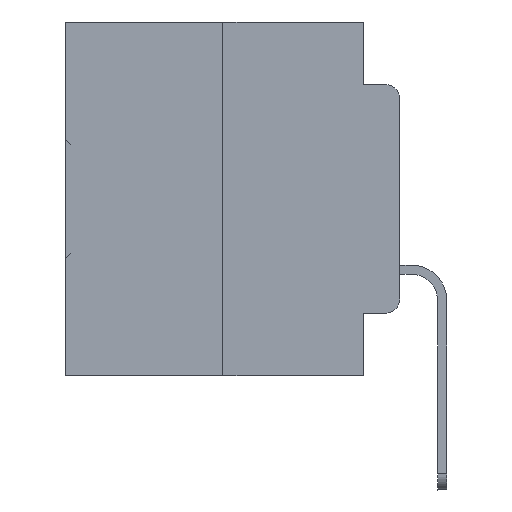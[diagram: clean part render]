
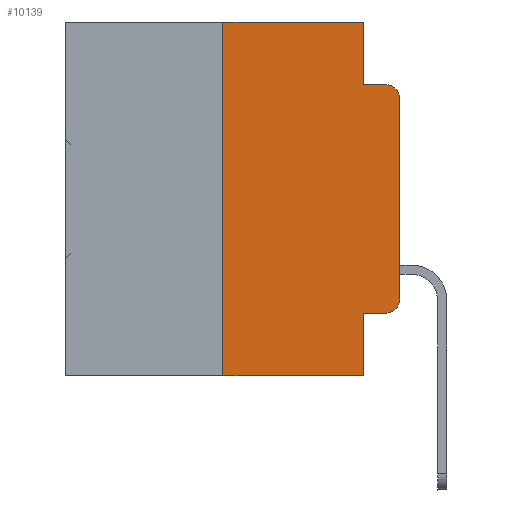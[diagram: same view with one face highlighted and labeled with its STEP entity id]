
A CAD part, left-side view. The second image highlights one B-rep face of the part: STEP entity #10139.
In plain terms, the highlighted planar face has unit normal (-1, 0, 0).
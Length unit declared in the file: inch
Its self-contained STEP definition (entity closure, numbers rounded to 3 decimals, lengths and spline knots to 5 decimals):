
#344 = VERTEX_POINT ( 'NONE', #29676 ) ;
#1409 = EDGE_CURVE ( 'NONE', #12813, #31002, #32425, .T. ) ;
#1522 = CARTESIAN_POINT ( 'NONE',  ( 0., 0., 0. ) ) ;
#1633 = CARTESIAN_POINT ( 'NONE',  ( 0., 0.051, -0.0885 ) ) ;
#2206 = LINE ( 'NONE', #34724, #25309 ) ;
#2281 = CARTESIAN_POINT ( 'NONE',  ( 0., 0.051, -0.4115 ) ) ;
#2851 = CARTESIAN_POINT ( 'NONE',  ( 0., 0.02, -0.1085 ) ) ;
#3725 = CARTESIAN_POINT ( 'NONE',  ( 0., 0.473, -0.5 ) ) ;
#4176 = CARTESIAN_POINT ( 'NONE',  ( 0., 0.02, -0.0885 ) ) ;
#4238 = PLANE ( 'NONE',  #6801 ) ;
#4602 = DIRECTION ( 'NONE',  ( 0., 0., -1. ) ) ;
#4656 = VECTOR ( 'NONE', #28134, 39.37008 ) ;
#5333 = DIRECTION ( 'NONE',  ( 0., 0., -1. ) ) ;
#5848 = EDGE_CURVE ( 'NONE', #8523, #9873, #6689, .T. ) ;
#6689 = LINE ( 'NONE', #14705, #17025 ) ;
#6700 = VECTOR ( 'NONE', #32070, 39.37008 ) ;
#6801 = AXIS2_PLACEMENT_3D ( 'NONE', #12415, #17924, #4602 ) ;
#7383 = LINE ( 'NONE', #1522, #31598 ) ;
#7455 = DIRECTION ( 'NONE',  ( -1., 0., 0. ) ) ;
#8523 = VERTEX_POINT ( 'NONE', #9254 ) ;
#9254 = CARTESIAN_POINT ( 'NONE',  ( 0., 0.051, 0. ) ) ;
#9873 = VERTEX_POINT ( 'NONE', #26986 ) ;
#9907 = CARTESIAN_POINT ( 'NONE',  ( 0., 0.473, 0. ) ) ;
#10139 = ADVANCED_FACE ( 'NONE', ( #28576 ), #4238, .F. ) ;
#10294 = CIRCLE ( 'NONE', #30708, 0.02 ) ;
#11257 = ORIENTED_EDGE ( 'NONE', *, *, #5848, .F. ) ;
#11300 = ORIENTED_EDGE ( 'NONE', *, *, #24654, .T. ) ;
#11871 = VERTEX_POINT ( 'NONE', #15208 ) ;
#12247 = ORIENTED_EDGE ( 'NONE', *, *, #19161, .F. ) ;
#12415 = CARTESIAN_POINT ( 'NONE',  ( 0., 0.473, 0. ) ) ;
#12483 = LINE ( 'NONE', #1633, #19912 ) ;
#12813 = VERTEX_POINT ( 'NONE', #2281 ) ;
#13400 = CARTESIAN_POINT ( 'NONE',  ( 0., 0.02, -0.4115 ) ) ;
#14019 = DIRECTION ( 'NONE',  ( -1., 0., 0. ) ) ;
#14705 = CARTESIAN_POINT ( 'NONE',  ( 0., 0.051, 0. ) ) ;
#14889 = CARTESIAN_POINT ( 'NONE',  ( 0., 0.051, -0.5 ) ) ;
#15131 = DIRECTION ( 'NONE',  ( 0., -1., 0. ) ) ;
#15208 = CARTESIAN_POINT ( 'NONE',  ( 0., 0.25, -0.5 ) ) ;
#15797 = CARTESIAN_POINT ( 'NONE',  ( 0., 0.02, -0.3915 ) ) ;
#16239 = CARTESIAN_POINT ( 'NONE',  ( 0., 0.051, -0.4115 ) ) ;
#16535 = EDGE_CURVE ( 'NONE', #9873, #20324, #12483, .T. ) ;
#16912 = EDGE_CURVE ( 'NONE', #344, #20324, #19348, .T. ) ;
#17009 = DIRECTION ( 'NONE',  ( 0., 0., -1. ) ) ;
#17025 = VECTOR ( 'NONE', #17009, 39.37008 ) ;
#17063 = LINE ( 'NONE', #3725, #20898 ) ;
#17924 = DIRECTION ( 'NONE',  ( 1., 0., 0. ) ) ;
#18304 = DIRECTION ( 'NONE',  ( 0., 0., -1. ) ) ;
#18483 = EDGE_CURVE ( 'NONE', #31002, #29661, #10294, .T. ) ;
#18798 = ORIENTED_EDGE ( 'NONE', *, *, #29195, .F. ) ;
#19161 = EDGE_CURVE ( 'NONE', #11871, #23018, #19989, .T. ) ;
#19348 = CIRCLE ( 'NONE', #29578, 0.02 ) ;
#19912 = VECTOR ( 'NONE', #15131, 39.37008 ) ;
#19989 = LINE ( 'NONE', #28512, #4656 ) ;
#20324 = VERTEX_POINT ( 'NONE', #4176 ) ;
#20685 = ORIENTED_EDGE ( 'NONE', *, *, #28958, .T. ) ;
#20898 = VECTOR ( 'NONE', #33598, 39.37008 ) ;
#21510 = ORIENTED_EDGE ( 'NONE', *, *, #22688, .F. ) ;
#22688 = EDGE_CURVE ( 'NONE', #12813, #29061, #2206, .T. ) ;
#23018 = VERTEX_POINT ( 'NONE', #25917 ) ;
#23525 = CARTESIAN_POINT ( 'NONE',  ( 0., 0., -0.3915 ) ) ;
#23570 = DIRECTION ( 'NONE',  ( 0., -1., 0. ) ) ;
#24654 = EDGE_CURVE ( 'NONE', #11871, #29061, #17063, .T. ) ;
#24675 = EDGE_LOOP ( 'NONE', ( #20685, #24939, #26715, #11257, #18798, #12247, #11300, #21510, #30266, #27965 ) ) ;
#24939 = ORIENTED_EDGE ( 'NONE', *, *, #16912, .T. ) ;
#25309 = VECTOR ( 'NONE', #29376, 39.37008 ) ;
#25917 = CARTESIAN_POINT ( 'NONE',  ( 0., 0.25, 0. ) ) ;
#26715 = ORIENTED_EDGE ( 'NONE', *, *, #16535, .F. ) ;
#26986 = CARTESIAN_POINT ( 'NONE',  ( 0., 0.051, -0.0885 ) ) ;
#27965 = ORIENTED_EDGE ( 'NONE', *, *, #18483, .T. ) ;
#28134 = DIRECTION ( 'NONE',  ( 0., 0., 1. ) ) ;
#28512 = CARTESIAN_POINT ( 'NONE',  ( 0., 0.25, 0. ) ) ;
#28576 = FACE_OUTER_BOUND ( 'NONE', #24675, .T. ) ;
#28958 = EDGE_CURVE ( 'NONE', #29661, #344, #7383, .T. ) ;
#29061 = VERTEX_POINT ( 'NONE', #14889 ) ;
#29063 = DIRECTION ( 'NONE',  ( 0., 0., 1. ) ) ;
#29195 = EDGE_CURVE ( 'NONE', #23018, #8523, #34241, .T. ) ;
#29376 = DIRECTION ( 'NONE',  ( 0., 0., -1. ) ) ;
#29578 = AXIS2_PLACEMENT_3D ( 'NONE', #2851, #14019, #5333 ) ;
#29661 = VERTEX_POINT ( 'NONE', #23525 ) ;
#29676 = CARTESIAN_POINT ( 'NONE',  ( 0., 0., -0.1085 ) ) ;
#30266 = ORIENTED_EDGE ( 'NONE', *, *, #1409, .T. ) ;
#30708 = AXIS2_PLACEMENT_3D ( 'NONE', #15797, #7455, #18304 ) ;
#31002 = VERTEX_POINT ( 'NONE', #13400 ) ;
#31054 = VECTOR ( 'NONE', #23570, 39.37008 ) ;
#31598 = VECTOR ( 'NONE', #29063, 39.37008 ) ;
#32070 = DIRECTION ( 'NONE',  ( 0., -1., 0. ) ) ;
#32425 = LINE ( 'NONE', #16239, #6700 ) ;
#33598 = DIRECTION ( 'NONE',  ( 0., -1., 0. ) ) ;
#34241 = LINE ( 'NONE', #9907, #31054 ) ;
#34724 = CARTESIAN_POINT ( 'NONE',  ( 0., 0.051, 0. ) ) ;
